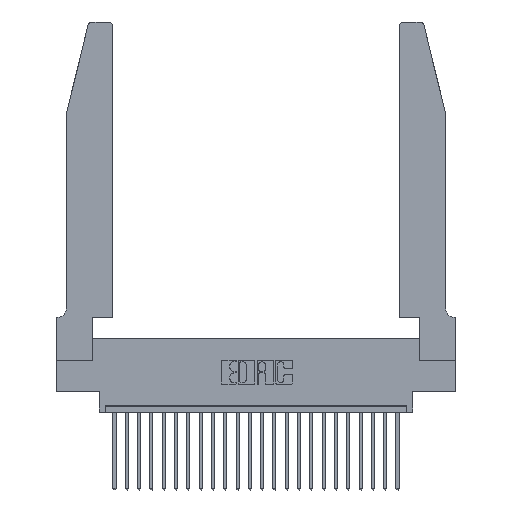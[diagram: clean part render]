
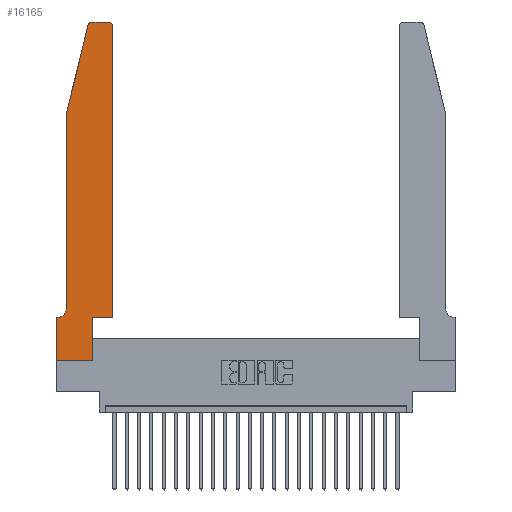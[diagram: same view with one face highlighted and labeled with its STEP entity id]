
A CAD part, top view. The second image highlights one B-rep face of the part: STEP entity #16165.
In plain terms, the highlighted planar face has unit normal (0, 0, 1).
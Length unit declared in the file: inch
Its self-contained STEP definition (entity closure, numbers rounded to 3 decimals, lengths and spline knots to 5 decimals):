
#20 = CARTESIAN_POINT ( 'NONE',  ( 0.4505, 0.35, 0.37 ) ) ;
#186 = EDGE_LOOP ( 'NONE', ( #3463, #3423, #9322, #7509, #1020, #19010, #6889, #2256, #16659, #16515, #13502, #19809 ) ) ;
#199 = EDGE_CURVE ( 'NONE', #20730, #4807, #15614, .T. ) ;
#651 = VERTEX_POINT ( 'NONE', #17824 ) ;
#1020 = ORIENTED_EDGE ( 'NONE', *, *, #13424, .T. ) ;
#1093 = EDGE_CURVE ( 'NONE', #10349, #651, #8819, .T. ) ;
#1164 = VECTOR ( 'NONE', #4888, 39.37008 ) ;
#1356 = EDGE_CURVE ( 'NONE', #15964, #10349, #17101, .T. ) ;
#1617 = VECTOR ( 'NONE', #23358, 39.37008 ) ;
#1722 = PLANE ( 'NONE',  #15625 ) ;
#1833 = VECTOR ( 'NONE', #2511, 39.37008 ) ;
#2104 = VECTOR ( 'NONE', #9944, 39.37008 ) ;
#2206 = VECTOR ( 'NONE', #12010, 39.37008 ) ;
#2256 = ORIENTED_EDGE ( 'NONE', *, *, #12052, .T. ) ;
#2439 = EDGE_CURVE ( 'NONE', #23435, #15964, #15492, .T. ) ;
#2511 = DIRECTION ( 'NONE',  ( 0., -1., 0. ) ) ;
#2684 = EDGE_CURVE ( 'NONE', #13582, #23435, #13315, .T. ) ;
#3423 = ORIENTED_EDGE ( 'NONE', *, *, #2439, .T. ) ;
#3463 = ORIENTED_EDGE ( 'NONE', *, *, #2684, .T. ) ;
#3527 = DIRECTION ( 'NONE',  ( 0., 0., 1. ) ) ;
#3971 = EDGE_CURVE ( 'NONE', #15345, #20730, #8051, .T. ) ;
#4190 = DIRECTION ( 'NONE',  ( -1., 0., 0. ) ) ;
#4592 = CARTESIAN_POINT ( 'NONE',  ( 0.2865, 0., 0.37 ) ) ;
#4807 = VERTEX_POINT ( 'NONE', #20550 ) ;
#4888 = DIRECTION ( 'NONE',  ( 0., -1., 0. ) ) ;
#5000 = DIRECTION ( 'NONE',  ( 1., 0., 0. ) ) ;
#5151 = DIRECTION ( 'NONE',  ( 0., 0., 1. ) ) ;
#5324 = CARTESIAN_POINT ( 'NONE',  ( 0.0755, 2., 0.37 ) ) ;
#5542 = EDGE_CURVE ( 'NONE', #9928, #20915, #20360, .T. ) ;
#5614 = AXIS2_PLACEMENT_3D ( 'NONE', #16883, #5151, #18887 ) ;
#6084 = LINE ( 'NONE', #15528, #2104 ) ;
#6222 = VECTOR ( 'NONE', #9927, 39.37008 ) ;
#6330 = EDGE_CURVE ( 'NONE', #12743, #24092, #19739, .T. ) ;
#6623 = AXIS2_PLACEMENT_3D ( 'NONE', #12753, #20815, #5000 ) ;
#6889 = ORIENTED_EDGE ( 'NONE', *, *, #199, .T. ) ;
#7457 = DIRECTION ( 'NONE',  ( 1., 0., 0. ) ) ;
#7509 = ORIENTED_EDGE ( 'NONE', *, *, #1093, .T. ) ;
#7607 = CARTESIAN_POINT ( 'NONE',  ( 0.0055, 0.35, 0.37 ) ) ;
#7680 = CIRCLE ( 'NONE', #6623, 0.03 ) ;
#8051 = LINE ( 'NONE', #15752, #6222 ) ;
#8499 = VECTOR ( 'NONE', #16079, 39.37008 ) ;
#8753 = CARTESIAN_POINT ( 'NONE',  ( 0.4205, 2.75, 0.37 ) ) ;
#8758 = DIRECTION ( 'NONE',  ( 0., 1., 0. ) ) ;
#8819 = LINE ( 'NONE', #22582, #1164 ) ;
#9322 = ORIENTED_EDGE ( 'NONE', *, *, #1356, .T. ) ;
#9695 = CIRCLE ( 'NONE', #12929, 0.07 ) ;
#9927 = DIRECTION ( 'NONE',  ( -1., 0., 0. ) ) ;
#9928 = VERTEX_POINT ( 'NONE', #4592 ) ;
#9944 = DIRECTION ( 'NONE',  ( 1., 0., 0. ) ) ;
#10349 = VERTEX_POINT ( 'NONE', #16908 ) ;
#11078 = CARTESIAN_POINT ( 'NONE',  ( 0.284, 2.75, 0.37 ) ) ;
#12010 = DIRECTION ( 'NONE',  ( 1., 0., 0. ) ) ;
#12052 = EDGE_CURVE ( 'NONE', #4807, #9928, #6084, .T. ) ;
#12743 = VERTEX_POINT ( 'NONE', #18851 ) ;
#12753 = CARTESIAN_POINT ( 'NONE',  ( 0.4205, 2.72, 0.37 ) ) ;
#12929 = AXIS2_PLACEMENT_3D ( 'NONE', #16186, #21979, #4190 ) ;
#13315 = LINE ( 'NONE', #16636, #21674 ) ;
#13424 = EDGE_CURVE ( 'NONE', #651, #15345, #9695, .T. ) ;
#13502 = ORIENTED_EDGE ( 'NONE', *, *, #6330, .T. ) ;
#13582 = VERTEX_POINT ( 'NONE', #8753 ) ;
#14255 = CARTESIAN_POINT ( 'NONE',  ( 0., 0., 0.37 ) ) ;
#15345 = VERTEX_POINT ( 'NONE', #7607 ) ;
#15492 = CIRCLE ( 'NONE', #5614, 0.03 ) ;
#15528 = CARTESIAN_POINT ( 'NONE',  ( 0., 0., 0.37 ) ) ;
#15614 = LINE ( 'NONE', #14255, #1833 ) ;
#15625 = AXIS2_PLACEMENT_3D ( 'NONE', #19405, #3527, #7457 ) ;
#15752 = CARTESIAN_POINT ( 'NONE',  ( 0.0755, 0.35, 0.37 ) ) ;
#15964 = VERTEX_POINT ( 'NONE', #23237 ) ;
#16079 = DIRECTION ( 'NONE',  ( -0.239, -0.971, 0. ) ) ;
#16165 = ADVANCED_FACE ( 'NONE', ( #24305 ), #1722, .T. ) ;
#16186 = CARTESIAN_POINT ( 'NONE',  ( 0.0055, 0.42, 0.37 ) ) ;
#16353 = VECTOR ( 'NONE', #8758, 39.37008 ) ;
#16515 = ORIENTED_EDGE ( 'NONE', *, *, #21258, .T. ) ;
#16636 = CARTESIAN_POINT ( 'NONE',  ( 0.2605, 2.75, 0.37 ) ) ;
#16659 = ORIENTED_EDGE ( 'NONE', *, *, #5542, .T. ) ;
#16883 = CARTESIAN_POINT ( 'NONE',  ( 0.284, 2.72, 0.37 ) ) ;
#16908 = CARTESIAN_POINT ( 'NONE',  ( 0.0755, 2., 0.37 ) ) ;
#16941 = LINE ( 'NONE', #19897, #2206 ) ;
#17101 = LINE ( 'NONE', #5324, #8499 ) ;
#17576 = EDGE_CURVE ( 'NONE', #24092, #13582, #7680, .T. ) ;
#17824 = CARTESIAN_POINT ( 'NONE',  ( 0.0755, 0.42, 0.37 ) ) ;
#17844 = CARTESIAN_POINT ( 'NONE',  ( 0., 0.35, 0.37 ) ) ;
#18632 = CARTESIAN_POINT ( 'NONE',  ( 0.2865, 0.35, 0.37 ) ) ;
#18826 = CARTESIAN_POINT ( 'NONE',  ( 0.2865, 0.35, 0.37 ) ) ;
#18851 = CARTESIAN_POINT ( 'NONE',  ( 0.4505, 0.35, 0.37 ) ) ;
#18887 = DIRECTION ( 'NONE',  ( 1., 0., 0. ) ) ;
#19010 = ORIENTED_EDGE ( 'NONE', *, *, #3971, .T. ) ;
#19405 = CARTESIAN_POINT ( 'NONE',  ( 0., 0.35, 0.37 ) ) ;
#19739 = LINE ( 'NONE', #20, #1617 ) ;
#19809 = ORIENTED_EDGE ( 'NONE', *, *, #17576, .T. ) ;
#19897 = CARTESIAN_POINT ( 'NONE',  ( 0.4505, 0.35, 0.37 ) ) ;
#20360 = LINE ( 'NONE', #18826, #16353 ) ;
#20550 = CARTESIAN_POINT ( 'NONE',  ( 0., 0., 0.37 ) ) ;
#20730 = VERTEX_POINT ( 'NONE', #17844 ) ;
#20815 = DIRECTION ( 'NONE',  ( 0., 0., 1. ) ) ;
#20915 = VERTEX_POINT ( 'NONE', #18632 ) ;
#21258 = EDGE_CURVE ( 'NONE', #20915, #12743, #16941, .T. ) ;
#21674 = VECTOR ( 'NONE', #24188, 39.37008 ) ;
#21979 = DIRECTION ( 'NONE',  ( 0., 0., -1. ) ) ;
#22582 = CARTESIAN_POINT ( 'NONE',  ( 0.0755, 2., 0.37 ) ) ;
#23237 = CARTESIAN_POINT ( 'NONE',  ( 0.25487, 2.72718, 0.37 ) ) ;
#23358 = DIRECTION ( 'NONE',  ( 0., 1., 0. ) ) ;
#23435 = VERTEX_POINT ( 'NONE', #11078 ) ;
#24092 = VERTEX_POINT ( 'NONE', #24268 ) ;
#24188 = DIRECTION ( 'NONE',  ( -1., 0., 0. ) ) ;
#24268 = CARTESIAN_POINT ( 'NONE',  ( 0.4505, 2.72, 0.37 ) ) ;
#24305 = FACE_OUTER_BOUND ( 'NONE', #186, .T. ) ;
